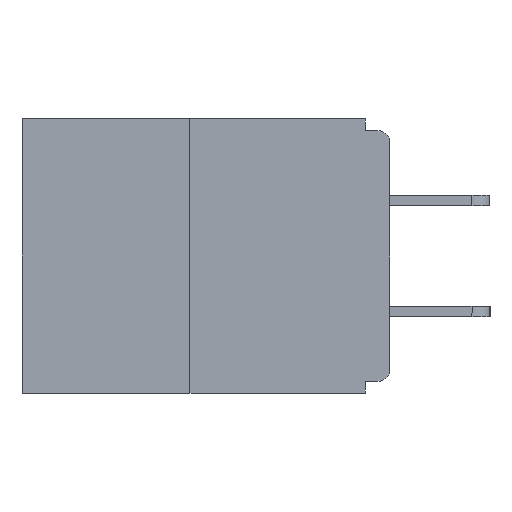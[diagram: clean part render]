
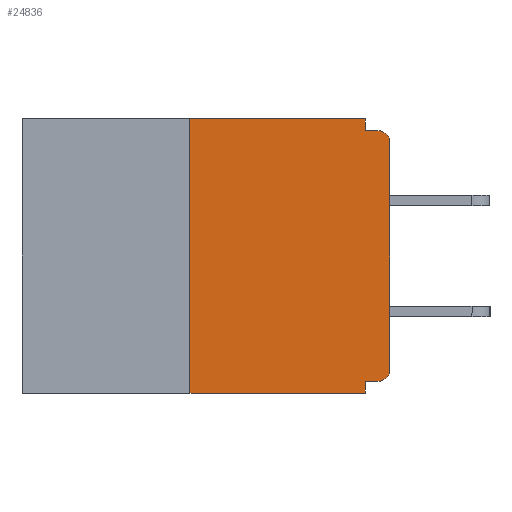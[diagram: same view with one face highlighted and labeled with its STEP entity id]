
A CAD part, left-side view. The second image highlights one B-rep face of the part: STEP entity #24836.
In plain terms, the highlighted planar face has unit normal (-1, 0, 0).
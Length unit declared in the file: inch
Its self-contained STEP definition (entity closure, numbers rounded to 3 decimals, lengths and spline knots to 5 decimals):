
#429 = DIRECTION ( 'NONE',  ( 0., 0., 1. ) ) ;
#615 = LINE ( 'NONE', #9557, #6664 ) ;
#631 = EDGE_CURVE ( 'NONE', #20136, #16345, #615, .T. ) ;
#1816 = CARTESIAN_POINT ( 'NONE',  ( 0., 0.015, -0.015 ) ) ;
#1973 = LINE ( 'NONE', #12721, #17476 ) ;
#2134 = CARTESIAN_POINT ( 'NONE',  ( 0., 0.25, -0.343 ) ) ;
#2204 = PLANE ( 'NONE',  #18971 ) ;
#2583 = ORIENTED_EDGE ( 'NONE', *, *, #631, .F. ) ;
#2609 = CARTESIAN_POINT ( 'NONE',  ( 0., 0.46, 0. ) ) ;
#2782 = DIRECTION ( 'NONE',  ( -1., 0., 0. ) ) ;
#2949 = DIRECTION ( 'NONE',  ( 0., -1., 0. ) ) ;
#3294 = VERTEX_POINT ( 'NONE', #11437 ) ;
#3770 = ORIENTED_EDGE ( 'NONE', *, *, #17111, .T. ) ;
#3865 = VECTOR ( 'NONE', #8223, 39.37008 ) ;
#4271 = VERTEX_POINT ( 'NONE', #1816 ) ;
#4704 = VECTOR ( 'NONE', #429, 39.37008 ) ;
#5016 = CARTESIAN_POINT ( 'NONE',  ( 0., 0.031, -0.343 ) ) ;
#5017 = DIRECTION ( 'NONE',  ( 0., -1., 0. ) ) ;
#5027 = CARTESIAN_POINT ( 'NONE',  ( 0., 0.015, -0.328 ) ) ;
#5121 = DIRECTION ( 'NONE',  ( 0., 0., -1. ) ) ;
#5174 = EDGE_CURVE ( 'NONE', #23367, #4271, #7167, .T. ) ;
#5451 = ORIENTED_EDGE ( 'NONE', *, *, #24885, .F. ) ;
#5481 = CARTESIAN_POINT ( 'NONE',  ( 0., 0., -0.03 ) ) ;
#5573 = DIRECTION ( 'NONE',  ( 0., 0., -1. ) ) ;
#5956 = EDGE_CURVE ( 'NONE', #20136, #7402, #19555, .T. ) ;
#6664 = VECTOR ( 'NONE', #23123, 39.37008 ) ;
#6864 = VECTOR ( 'NONE', #2949, 39.37008 ) ;
#7167 = CIRCLE ( 'NONE', #8539, 0.015 ) ;
#7402 = VERTEX_POINT ( 'NONE', #8147 ) ;
#7445 = DIRECTION ( 'NONE',  ( -1., 0., 0. ) ) ;
#8147 = CARTESIAN_POINT ( 'NONE',  ( 0., 0., -0.313 ) ) ;
#8223 = DIRECTION ( 'NONE',  ( 0., 0., 1. ) ) ;
#8335 = EDGE_CURVE ( 'NONE', #12195, #4271, #8722, .T. ) ;
#8384 = DIRECTION ( 'NONE',  ( 0., 0., -1. ) ) ;
#8539 = AXIS2_PLACEMENT_3D ( 'NONE', #15453, #7445, #5573 ) ;
#8638 = VERTEX_POINT ( 'NONE', #5016 ) ;
#8722 = LINE ( 'NONE', #20905, #20899 ) ;
#9142 = CARTESIAN_POINT ( 'NONE',  ( 0., 0.031, 0. ) ) ;
#9355 = DIRECTION ( 'NONE',  ( 0., -1., 0. ) ) ;
#9557 = CARTESIAN_POINT ( 'NONE',  ( 0., 0., -0.328 ) ) ;
#10842 = EDGE_LOOP ( 'NONE', ( #5451, #15325, #3770, #11753, #2583, #17894, #11700, #21774, #20002, #25070 ) ) ;
#11123 = LINE ( 'NONE', #15883, #3865 ) ;
#11317 = LINE ( 'NONE', #22306, #20426 ) ;
#11392 = VERTEX_POINT ( 'NONE', #2134 ) ;
#11437 = CARTESIAN_POINT ( 'NONE',  ( 0., 0.25, 0. ) ) ;
#11700 = ORIENTED_EDGE ( 'NONE', *, *, #13800, .T. ) ;
#11753 = ORIENTED_EDGE ( 'NONE', *, *, #14884, .F. ) ;
#12195 = VERTEX_POINT ( 'NONE', #24460 ) ;
#12229 = CARTESIAN_POINT ( 'NONE',  ( 0., 0.46, 0. ) ) ;
#12235 = CARTESIAN_POINT ( 'NONE',  ( 0., 0.015, -0.313 ) ) ;
#12650 = DIRECTION ( 'NONE',  ( 0., 0., -1. ) ) ;
#12721 = CARTESIAN_POINT ( 'NONE',  ( 0., 0.031, -0.343 ) ) ;
#13309 = VECTOR ( 'NONE', #5121, 39.37008 ) ;
#13551 = LINE ( 'NONE', #17846, #4704 ) ;
#13800 = EDGE_CURVE ( 'NONE', #7402, #23367, #11123, .T. ) ;
#14653 = EDGE_CURVE ( 'NONE', #11392, #3294, #13551, .T. ) ;
#14884 = EDGE_CURVE ( 'NONE', #16345, #8638, #1973, .T. ) ;
#14971 = VERTEX_POINT ( 'NONE', #9142 ) ;
#15325 = ORIENTED_EDGE ( 'NONE', *, *, #14653, .F. ) ;
#15453 = CARTESIAN_POINT ( 'NONE',  ( 0., 0.015, -0.03 ) ) ;
#15883 = CARTESIAN_POINT ( 'NONE',  ( 0., 0., 0. ) ) ;
#16223 = AXIS2_PLACEMENT_3D ( 'NONE', #12235, #2782, #16290 ) ;
#16290 = DIRECTION ( 'NONE',  ( 0., 0., -1. ) ) ;
#16308 = LINE ( 'NONE', #2609, #6864 ) ;
#16345 = VERTEX_POINT ( 'NONE', #20782 ) ;
#17111 = EDGE_CURVE ( 'NONE', #11392, #8638, #11317, .T. ) ;
#17476 = VECTOR ( 'NONE', #12650, 39.37008 ) ;
#17846 = CARTESIAN_POINT ( 'NONE',  ( 0., 0.25, 0. ) ) ;
#17894 = ORIENTED_EDGE ( 'NONE', *, *, #5956, .T. ) ;
#18971 = AXIS2_PLACEMENT_3D ( 'NONE', #12229, #20033, #8384 ) ;
#19555 = CIRCLE ( 'NONE', #16223, 0.015 ) ;
#19707 = LINE ( 'NONE', #20737, #13309 ) ;
#20002 = ORIENTED_EDGE ( 'NONE', *, *, #8335, .F. ) ;
#20033 = DIRECTION ( 'NONE',  ( 1., 0., 0. ) ) ;
#20136 = VERTEX_POINT ( 'NONE', #5027 ) ;
#20426 = VECTOR ( 'NONE', #5017, 39.37008 ) ;
#20572 = FACE_OUTER_BOUND ( 'NONE', #10842, .T. ) ;
#20737 = CARTESIAN_POINT ( 'NONE',  ( 0., 0.031, 0. ) ) ;
#20782 = CARTESIAN_POINT ( 'NONE',  ( 0., 0.031, -0.328 ) ) ;
#20899 = VECTOR ( 'NONE', #9355, 39.37008 ) ;
#20905 = CARTESIAN_POINT ( 'NONE',  ( 0., 0., -0.015 ) ) ;
#21774 = ORIENTED_EDGE ( 'NONE', *, *, #5174, .T. ) ;
#22306 = CARTESIAN_POINT ( 'NONE',  ( 0., 0.46, -0.343 ) ) ;
#23123 = DIRECTION ( 'NONE',  ( 0., 1., 0. ) ) ;
#23367 = VERTEX_POINT ( 'NONE', #5481 ) ;
#23920 = EDGE_CURVE ( 'NONE', #14971, #12195, #19707, .T. ) ;
#24460 = CARTESIAN_POINT ( 'NONE',  ( 0., 0.031, -0.015 ) ) ;
#24836 = ADVANCED_FACE ( 'NONE', ( #20572 ), #2204, .F. ) ;
#24885 = EDGE_CURVE ( 'NONE', #3294, #14971, #16308, .T. ) ;
#25070 = ORIENTED_EDGE ( 'NONE', *, *, #23920, .F. ) ;
